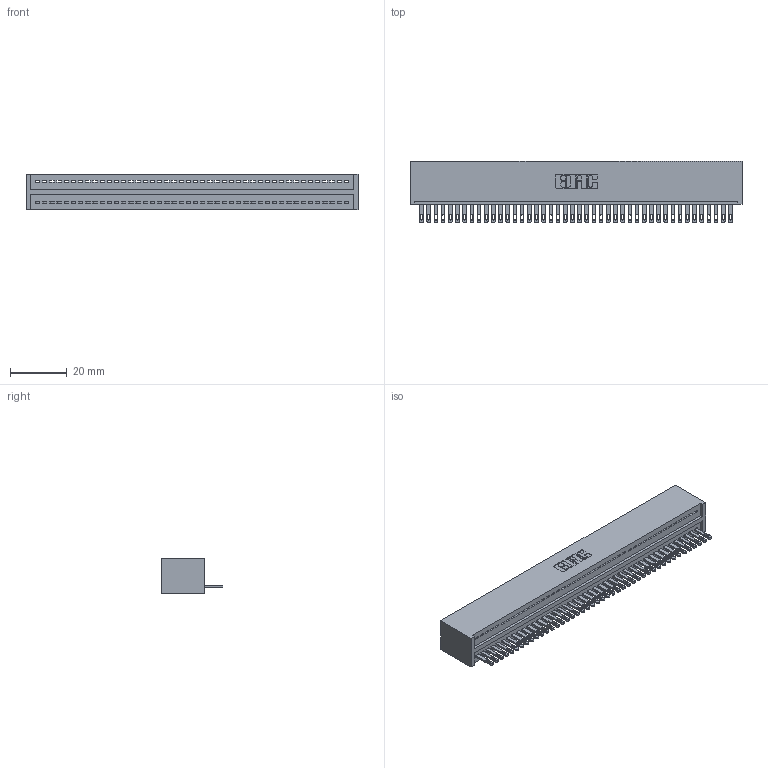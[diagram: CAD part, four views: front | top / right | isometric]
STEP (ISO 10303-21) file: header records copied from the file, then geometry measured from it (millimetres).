
FILE_DESCRIPTION (( 'STEP AP203' ), '1' );
FILE_NAME ('325-044-500-101.STEP', '2020-02-24T22:15:10', ( '' ), ( '' ), 'SwSTEP 2.0', 'SolidWorks 2016', '' );
FILE_SCHEMA (( 'CONFIG_CONTROL_DESIGN' ));
Length unit declared in the file: inch
Products named in the file (3): 325-044-500-101; 325 Part_Lugless; 325-292-001_325-293-100
Assembly tree (45 placements, depth 2):
  325-044-500-101
    325 Part_Lugless
    325-292-001_325-293-100  x44
Bounding box: 117.4 x 21.84 x 12.45 mm (x, y, z)
Volume: 15518.5 mm3; surface area: 17581.3 mm2
Topology: 45 solids, 45 shells, 2482 faces, 7679 edges, 5118 vertices
Faces by surface type: plane 1650, cylinder 832
Entity records: 26293 total; most frequent: CARTESIAN_POINT 4542, ORIENTED_EDGE 4522, DIRECTION 3821, EDGE_CURVE 2261, LINE 2137, VECTOR 2137, VERTEX_POINT 1506, AXIS2_PLACEMENT_3D 842
